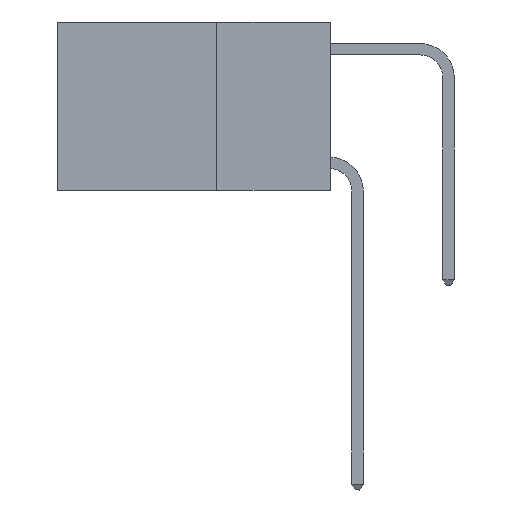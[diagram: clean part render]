
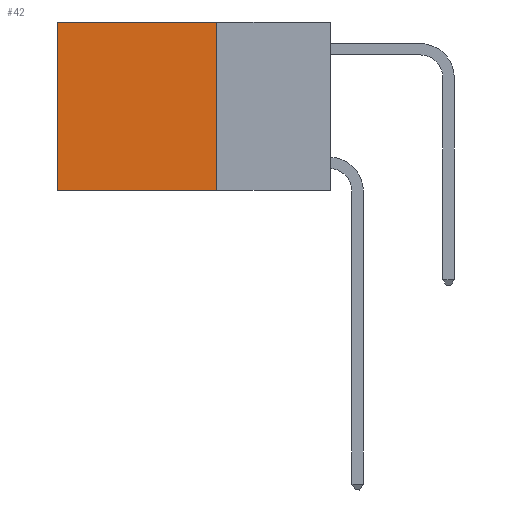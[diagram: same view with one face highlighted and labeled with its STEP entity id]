
A CAD part, left-side view. The second image highlights one B-rep face of the part: STEP entity #42.
In plain terms, the highlighted planar face has unit normal (-1, 0, 0).
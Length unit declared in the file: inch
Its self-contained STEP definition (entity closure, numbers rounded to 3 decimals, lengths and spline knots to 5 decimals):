
#42 = ADVANCED_FACE ( 'NONE', ( #12776 ), #11151, .F. ) ;
#358 = CARTESIAN_POINT ( 'NONE',  ( 0.2625, 0.25, -0.37 ) ) ;
#680 = EDGE_CURVE ( 'NONE', #12605, #2050, #16143, .T. ) ;
#913 = EDGE_LOOP ( 'NONE', ( #6410, #8267, #7112, #9637 ) ) ;
#1048 = DIRECTION ( 'NONE',  ( 0., 0., -1. ) ) ;
#1145 = DIRECTION ( 'NONE',  ( 0., 1., 0. ) ) ;
#2050 = VERTEX_POINT ( 'NONE', #358 ) ;
#2270 = EDGE_CURVE ( 'NONE', #2050, #14257, #7752, .T. ) ;
#2861 = VECTOR ( 'NONE', #12364, 39.37008 ) ;
#4681 = CARTESIAN_POINT ( 'NONE',  ( 0.2625, 0.25, 0. ) ) ;
#5652 = VERTEX_POINT ( 'NONE', #15509 ) ;
#6199 = DIRECTION ( 'NONE',  ( 1., 0., 0. ) ) ;
#6410 = ORIENTED_EDGE ( 'NONE', *, *, #11735, .T. ) ;
#7039 = DIRECTION ( 'NONE',  ( 0., 1., 0. ) ) ;
#7112 = ORIENTED_EDGE ( 'NONE', *, *, #680, .F. ) ;
#7425 = VECTOR ( 'NONE', #14133, 39.37008 ) ;
#7661 = CARTESIAN_POINT ( 'NONE',  ( 0.2625, 0.25, 0. ) ) ;
#7752 = LINE ( 'NONE', #11673, #16351 ) ;
#8267 = ORIENTED_EDGE ( 'NONE', *, *, #2270, .F. ) ;
#8977 = CARTESIAN_POINT ( 'NONE',  ( 0.2625, 0.6, 0. ) ) ;
#9545 = CARTESIAN_POINT ( 'NONE',  ( 0.2625, 0.6, -0.37 ) ) ;
#9548 = LINE ( 'NONE', #9625, #15124 ) ;
#9625 = CARTESIAN_POINT ( 'NONE',  ( 0.2625, 0.25, 0. ) ) ;
#9637 = ORIENTED_EDGE ( 'NONE', *, *, #15613, .T. ) ;
#9701 = CARTESIAN_POINT ( 'NONE',  ( 0.2625, 0.25, 0. ) ) ;
#11151 = PLANE ( 'NONE',  #11839 ) ;
#11673 = CARTESIAN_POINT ( 'NONE',  ( 0.2625, 0.25, -0.37 ) ) ;
#11735 = EDGE_CURVE ( 'NONE', #5652, #14257, #15273, .T. ) ;
#11839 = AXIS2_PLACEMENT_3D ( 'NONE', #7661, #6199, #1048 ) ;
#12364 = DIRECTION ( 'NONE',  ( 0., 0., -1. ) ) ;
#12605 = VERTEX_POINT ( 'NONE', #9701 ) ;
#12776 = FACE_OUTER_BOUND ( 'NONE', #913, .T. ) ;
#14133 = DIRECTION ( 'NONE',  ( 0., 0., -1. ) ) ;
#14257 = VERTEX_POINT ( 'NONE', #9545 ) ;
#15124 = VECTOR ( 'NONE', #7039, 39.37008 ) ;
#15273 = LINE ( 'NONE', #8977, #7425 ) ;
#15509 = CARTESIAN_POINT ( 'NONE',  ( 0.2625, 0.6, 0. ) ) ;
#15613 = EDGE_CURVE ( 'NONE', #12605, #5652, #9548, .T. ) ;
#16143 = LINE ( 'NONE', #4681, #2861 ) ;
#16351 = VECTOR ( 'NONE', #1145, 39.37008 ) ;
